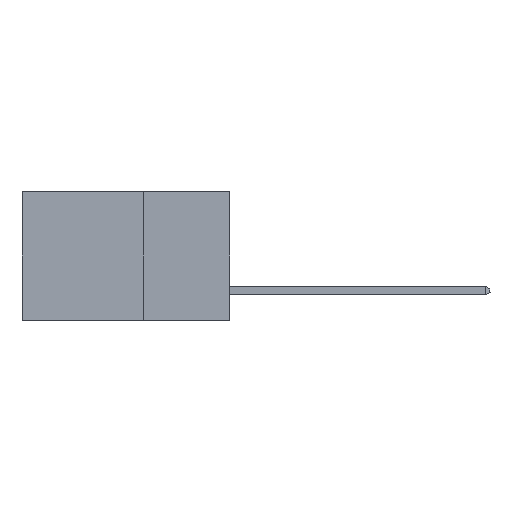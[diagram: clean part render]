
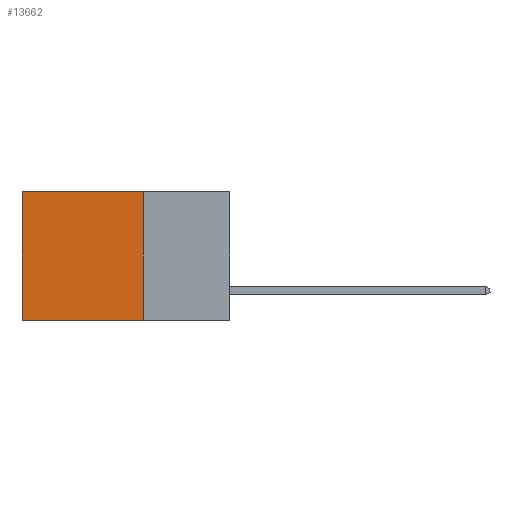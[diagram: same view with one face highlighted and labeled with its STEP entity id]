
A CAD part, left-side view. The second image highlights one B-rep face of the part: STEP entity #13662.
In plain terms, the highlighted planar face has unit normal (-1, 0, 0).
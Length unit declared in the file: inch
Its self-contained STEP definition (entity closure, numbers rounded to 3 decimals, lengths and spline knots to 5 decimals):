
#86 = CARTESIAN_POINT ( 'NONE',  ( 0.298, 0.6, -0.37 ) ) ;
#319 = FACE_OUTER_BOUND ( 'NONE', #18325, .T. ) ;
#324 = EDGE_CURVE ( 'NONE', #2741, #3400, #20540, .T. ) ;
#1408 = EDGE_CURVE ( 'NONE', #2741, #1892, #19450, .T. ) ;
#1892 = VERTEX_POINT ( 'NONE', #12836 ) ;
#2741 = VERTEX_POINT ( 'NONE', #9023 ) ;
#2957 = LINE ( 'NONE', #10347, #16542 ) ;
#3115 = EDGE_CURVE ( 'NONE', #3400, #4090, #2957, .T. ) ;
#3304 = ORIENTED_EDGE ( 'NONE', *, *, #324, .F. ) ;
#3400 = VERTEX_POINT ( 'NONE', #9742 ) ;
#4090 = VERTEX_POINT ( 'NONE', #86 ) ;
#4099 = PLANE ( 'NONE',  #13572 ) ;
#4243 = VECTOR ( 'NONE', #10667, 39.37008 ) ;
#5584 = ORIENTED_EDGE ( 'NONE', *, *, #1408, .T. ) ;
#5815 = DIRECTION ( 'NONE',  ( 0., 0., -1. ) ) ;
#5935 = DIRECTION ( 'NONE',  ( 0., 0., -1. ) ) ;
#6429 = CARTESIAN_POINT ( 'NONE',  ( 0.298, 0.25, 0. ) ) ;
#7440 = EDGE_CURVE ( 'NONE', #1892, #4090, #15603, .T. ) ;
#9023 = CARTESIAN_POINT ( 'NONE',  ( 0.298, 0.25, 0. ) ) ;
#9601 = DIRECTION ( 'NONE',  ( 0., 0., -1. ) ) ;
#9742 = CARTESIAN_POINT ( 'NONE',  ( 0.298, 0.25, -0.37 ) ) ;
#10347 = CARTESIAN_POINT ( 'NONE',  ( 0.298, 0.25, -0.37 ) ) ;
#10667 = DIRECTION ( 'NONE',  ( 0., 1., 0. ) ) ;
#11001 = DIRECTION ( 'NONE',  ( 1., 0., 0. ) ) ;
#12549 = CARTESIAN_POINT ( 'NONE',  ( 0.298, 0.6, 0. ) ) ;
#12836 = CARTESIAN_POINT ( 'NONE',  ( 0.298, 0.6, 0. ) ) ;
#13093 = VECTOR ( 'NONE', #9601, 39.37008 ) ;
#13572 = AXIS2_PLACEMENT_3D ( 'NONE', #21205, #11001, #5815 ) ;
#13662 = ADVANCED_FACE ( 'NONE', ( #319 ), #4099, .F. ) ;
#13717 = VECTOR ( 'NONE', #5935, 39.37008 ) ;
#13887 = DIRECTION ( 'NONE',  ( 0., 1., 0. ) ) ;
#15585 = ORIENTED_EDGE ( 'NONE', *, *, #3115, .F. ) ;
#15603 = LINE ( 'NONE', #12549, #13717 ) ;
#15743 = ORIENTED_EDGE ( 'NONE', *, *, #7440, .T. ) ;
#16542 = VECTOR ( 'NONE', #13887, 39.37008 ) ;
#18325 = EDGE_LOOP ( 'NONE', ( #15743, #15585, #3304, #5584 ) ) ;
#19450 = LINE ( 'NONE', #20870, #4243 ) ;
#20540 = LINE ( 'NONE', #6429, #13093 ) ;
#20870 = CARTESIAN_POINT ( 'NONE',  ( 0.298, 0.25, 0. ) ) ;
#21205 = CARTESIAN_POINT ( 'NONE',  ( 0.298, 0.25, 0. ) ) ;
